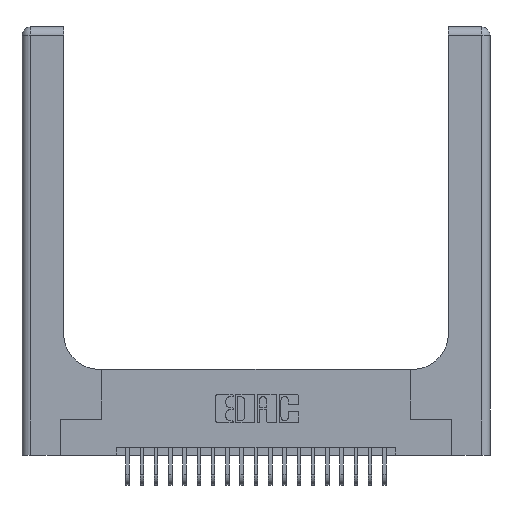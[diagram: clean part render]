
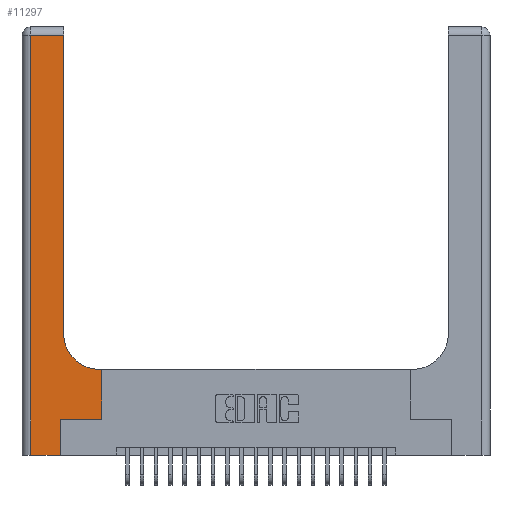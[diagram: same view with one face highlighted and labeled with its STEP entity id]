
A CAD part, top view. The second image highlights one B-rep face of the part: STEP entity #11297.
In plain terms, the highlighted planar face has unit normal (0, 0, 1).
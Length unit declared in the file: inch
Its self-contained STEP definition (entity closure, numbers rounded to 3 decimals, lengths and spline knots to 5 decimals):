
#247 = ORIENTED_EDGE ( 'NONE', *, *, #20534, .T. ) ;
#874 = VERTEX_POINT ( 'NONE', #17636 ) ;
#1968 = ORIENTED_EDGE ( 'NONE', *, *, #13938, .T. ) ;
#2499 = CARTESIAN_POINT ( 'NONE',  ( 0.2915, 0.6, 0.37 ) ) ;
#2767 = CARTESIAN_POINT ( 'NONE',  ( 0.2915, 0.85, 0.37 ) ) ;
#3060 = CARTESIAN_POINT ( 'NONE',  ( 0.06, 2.94, 0.37 ) ) ;
#3197 = CARTESIAN_POINT ( 'NONE',  ( 0.269, 0.25, 0.37 ) ) ;
#3322 = DIRECTION ( 'NONE',  ( 0., 1., 0. ) ) ;
#3428 = CARTESIAN_POINT ( 'NONE',  ( 0.269, 0., 0.37 ) ) ;
#3624 = CARTESIAN_POINT ( 'NONE',  ( 0.269, 0., 0.37 ) ) ;
#4014 = LINE ( 'NONE', #4786, #23832 ) ;
#4416 = CARTESIAN_POINT ( 'NONE',  ( 0., 2.94, 0.37 ) ) ;
#4433 = DIRECTION ( 'NONE',  ( -1., 0., 0. ) ) ;
#4492 = DIRECTION ( 'NONE',  ( -1., 0., 0. ) ) ;
#4786 = CARTESIAN_POINT ( 'NONE',  ( 0.5585, 0.25, 0.37 ) ) ;
#5119 = LINE ( 'NONE', #24378, #24324 ) ;
#6238 = EDGE_CURVE ( 'NONE', #21259, #20198, #23138, .T. ) ;
#6254 = DIRECTION ( 'NONE',  ( 1., 0., 0. ) ) ;
#6633 = LINE ( 'NONE', #9949, #19013 ) ;
#7023 = DIRECTION ( 'NONE',  ( 0., -1., 0. ) ) ;
#7319 = EDGE_CURVE ( 'NONE', #874, #24090, #13703, .T. ) ;
#7427 = PLANE ( 'NONE',  #24239 ) ;
#7901 = VECTOR ( 'NONE', #7023, 39.37008 ) ;
#7906 = DIRECTION ( 'NONE',  ( 1., 0., 0. ) ) ;
#8593 = CARTESIAN_POINT ( 'NONE',  ( 0.5415, 0.85, 0.37 ) ) ;
#8710 = VERTEX_POINT ( 'NONE', #3060 ) ;
#9077 = LINE ( 'NONE', #10203, #23678 ) ;
#9949 = CARTESIAN_POINT ( 'NONE',  ( 0.269, 0.25, 0.37 ) ) ;
#10203 = CARTESIAN_POINT ( 'NONE',  ( 0., 0., 0.37 ) ) ;
#10334 = ORIENTED_EDGE ( 'NONE', *, *, #20776, .T. ) ;
#10548 = DIRECTION ( 'NONE',  ( 1., 0., 0. ) ) ;
#10700 = ORIENTED_EDGE ( 'NONE', *, *, #10942, .T. ) ;
#10942 = EDGE_CURVE ( 'NONE', #16442, #874, #15048, .T. ) ;
#11297 = ADVANCED_FACE ( 'NONE', ( #21848 ), #7427, .F. ) ;
#11365 = DIRECTION ( 'NONE',  ( 0., 0., -1. ) ) ;
#11633 = CARTESIAN_POINT ( 'NONE',  ( 0.5585, 0.25, 0.37 ) ) ;
#11711 = CARTESIAN_POINT ( 'NONE',  ( 0.2915, 2.94, 0.37 ) ) ;
#12375 = EDGE_LOOP ( 'NONE', ( #247, #16509, #12472, #17837, #18375, #10334, #1968, #10700, #15246 ) ) ;
#12472 = ORIENTED_EDGE ( 'NONE', *, *, #20177, .T. ) ;
#12629 = DIRECTION ( 'NONE',  ( 0., 1., 0. ) ) ;
#12721 = VECTOR ( 'NONE', #4492, 39.37008 ) ;
#13045 = AXIS2_PLACEMENT_3D ( 'NONE', #8593, #21974, #10548 ) ;
#13703 = CIRCLE ( 'NONE', #13045, 0.25 ) ;
#13938 = EDGE_CURVE ( 'NONE', #16711, #16442, #4014, .T. ) ;
#14441 = VECTOR ( 'NONE', #4433, 39.37008 ) ;
#15048 = LINE ( 'NONE', #2499, #14441 ) ;
#15246 = ORIENTED_EDGE ( 'NONE', *, *, #7319, .T. ) ;
#16442 = VERTEX_POINT ( 'NONE', #22239 ) ;
#16509 = ORIENTED_EDGE ( 'NONE', *, *, #17474, .T. ) ;
#16711 = VERTEX_POINT ( 'NONE', #11633 ) ;
#17411 = VERTEX_POINT ( 'NONE', #21523 ) ;
#17474 = EDGE_CURVE ( 'NONE', #24425, #8710, #17811, .T. ) ;
#17636 = CARTESIAN_POINT ( 'NONE',  ( 0.5415, 0.6, 0.37 ) ) ;
#17811 = LINE ( 'NONE', #4416, #12721 ) ;
#17837 = ORIENTED_EDGE ( 'NONE', *, *, #18119, .T. ) ;
#18119 = EDGE_CURVE ( 'NONE', #17411, #21259, #9077, .T. ) ;
#18375 = ORIENTED_EDGE ( 'NONE', *, *, #6238, .T. ) ;
#19013 = VECTOR ( 'NONE', #7906, 39.37008 ) ;
#20177 = EDGE_CURVE ( 'NONE', #8710, #17411, #23750, .T. ) ;
#20198 = VERTEX_POINT ( 'NONE', #3197 ) ;
#20497 = CARTESIAN_POINT ( 'NONE',  ( 0.06, 3., 0.37 ) ) ;
#20534 = EDGE_CURVE ( 'NONE', #24090, #24425, #5119, .T. ) ;
#20776 = EDGE_CURVE ( 'NONE', #20198, #16711, #6633, .T. ) ;
#20792 = CARTESIAN_POINT ( 'NONE',  ( 0., 3., 0.37 ) ) ;
#21259 = VERTEX_POINT ( 'NONE', #3624 ) ;
#21523 = CARTESIAN_POINT ( 'NONE',  ( 0.06, 0., 0.37 ) ) ;
#21848 = FACE_OUTER_BOUND ( 'NONE', #12375, .T. ) ;
#21974 = DIRECTION ( 'NONE',  ( 0., 0., -1. ) ) ;
#22239 = CARTESIAN_POINT ( 'NONE',  ( 0.5585, 0.6, 0.37 ) ) ;
#22556 = VECTOR ( 'NONE', #22692, 39.37008 ) ;
#22692 = DIRECTION ( 'NONE',  ( 0., 1., 0. ) ) ;
#23138 = LINE ( 'NONE', #3428, #22556 ) ;
#23678 = VECTOR ( 'NONE', #6254, 39.37008 ) ;
#23750 = LINE ( 'NONE', #20497, #7901 ) ;
#23832 = VECTOR ( 'NONE', #12629, 39.37008 ) ;
#24090 = VERTEX_POINT ( 'NONE', #2767 ) ;
#24239 = AXIS2_PLACEMENT_3D ( 'NONE', #20792, #11365, #24645 ) ;
#24324 = VECTOR ( 'NONE', #3322, 39.37008 ) ;
#24378 = CARTESIAN_POINT ( 'NONE',  ( 0.2915, 3., 0.37 ) ) ;
#24425 = VERTEX_POINT ( 'NONE', #11711 ) ;
#24645 = DIRECTION ( 'NONE',  ( -1., 0., 0. ) ) ;
